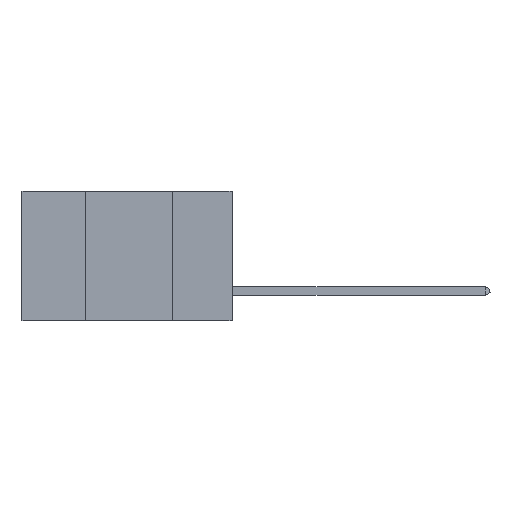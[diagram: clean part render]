
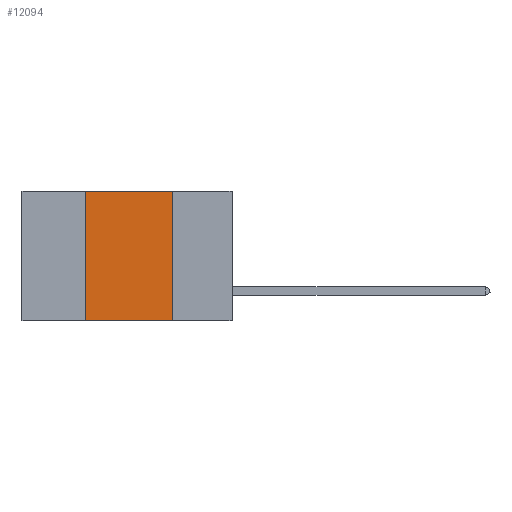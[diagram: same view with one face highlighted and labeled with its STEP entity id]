
A CAD part, left-side view. The second image highlights one B-rep face of the part: STEP entity #12094.
In plain terms, the highlighted planar face has unit normal (-1, 0, 0).
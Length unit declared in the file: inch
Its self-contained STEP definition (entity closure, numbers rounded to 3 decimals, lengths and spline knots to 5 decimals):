
#1949 = VERTEX_POINT ( 'NONE', #13437 ) ;
#2941 = DIRECTION ( 'NONE',  ( 1., 0., 0. ) ) ;
#4135 = VERTEX_POINT ( 'NONE', #6516 ) ;
#4414 = CARTESIAN_POINT ( 'NONE',  ( 0., 0.17, 0. ) ) ;
#4962 = EDGE_CURVE ( 'NONE', #1949, #4135, #7468, .T. ) ;
#5593 = LINE ( 'NONE', #12848, #19812 ) ;
#5698 = LINE ( 'NONE', #12471, #15815 ) ;
#6486 = ORIENTED_EDGE ( 'NONE', *, *, #13995, .F. ) ;
#6502 = VERTEX_POINT ( 'NONE', #23247 ) ;
#6516 = CARTESIAN_POINT ( 'NONE',  ( 0., 0.17, -0.37 ) ) ;
#6821 = DIRECTION ( 'NONE',  ( 0., 0., 1. ) ) ;
#6840 = DIRECTION ( 'NONE',  ( 0., 0., -1. ) ) ;
#6892 = CARTESIAN_POINT ( 'NONE',  ( 0., 0.6, 0. ) ) ;
#7342 = CARTESIAN_POINT ( 'NONE',  ( 0., 0.6, -0.37 ) ) ;
#7468 = LINE ( 'NONE', #7342, #19171 ) ;
#8254 = VERTEX_POINT ( 'NONE', #4414 ) ;
#8427 = LINE ( 'NONE', #15212, #13461 ) ;
#9802 = FACE_OUTER_BOUND ( 'NONE', #18827, .T. ) ;
#10585 = ORIENTED_EDGE ( 'NONE', *, *, #4962, .T. ) ;
#11138 = DIRECTION ( 'NONE',  ( 0., 0., -1. ) ) ;
#11594 = DIRECTION ( 'NONE',  ( 0., -1., 0. ) ) ;
#12094 = ADVANCED_FACE ( 'NONE', ( #9802 ), #19018, .F. ) ;
#12471 = CARTESIAN_POINT ( 'NONE',  ( 0., 0.6, 0. ) ) ;
#12848 = CARTESIAN_POINT ( 'NONE',  ( 0., 0.17, 0. ) ) ;
#13437 = CARTESIAN_POINT ( 'NONE',  ( 0., 0.42, -0.37 ) ) ;
#13461 = VECTOR ( 'NONE', #6821, 39.37008 ) ;
#13995 = EDGE_CURVE ( 'NONE', #1949, #6502, #8427, .T. ) ;
#15212 = CARTESIAN_POINT ( 'NONE',  ( 0., 0.42, 0. ) ) ;
#15815 = VECTOR ( 'NONE', #22793, 39.37008 ) ;
#16892 = EDGE_CURVE ( 'NONE', #6502, #8254, #5698, .T. ) ;
#17715 = ORIENTED_EDGE ( 'NONE', *, *, #16892, .F. ) ;
#18428 = EDGE_CURVE ( 'NONE', #8254, #4135, #5593, .T. ) ;
#18827 = EDGE_LOOP ( 'NONE', ( #23067, #17715, #6486, #10585 ) ) ;
#19018 = PLANE ( 'NONE',  #23895 ) ;
#19171 = VECTOR ( 'NONE', #11594, 39.37008 ) ;
#19812 = VECTOR ( 'NONE', #6840, 39.37008 ) ;
#22793 = DIRECTION ( 'NONE',  ( 0., -1., 0. ) ) ;
#23067 = ORIENTED_EDGE ( 'NONE', *, *, #18428, .F. ) ;
#23247 = CARTESIAN_POINT ( 'NONE',  ( 0., 0.42, 0. ) ) ;
#23895 = AXIS2_PLACEMENT_3D ( 'NONE', #6892, #2941, #11138 ) ;
